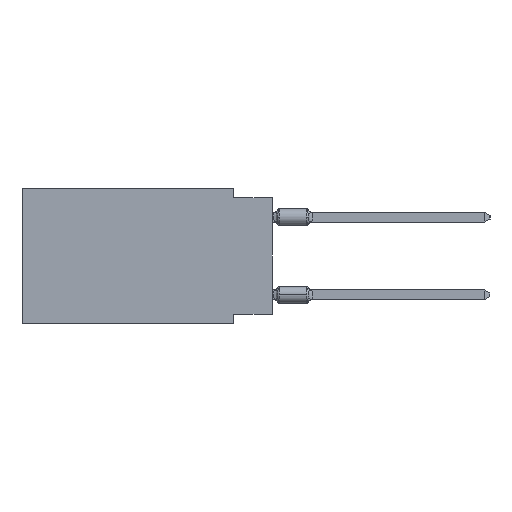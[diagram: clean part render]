
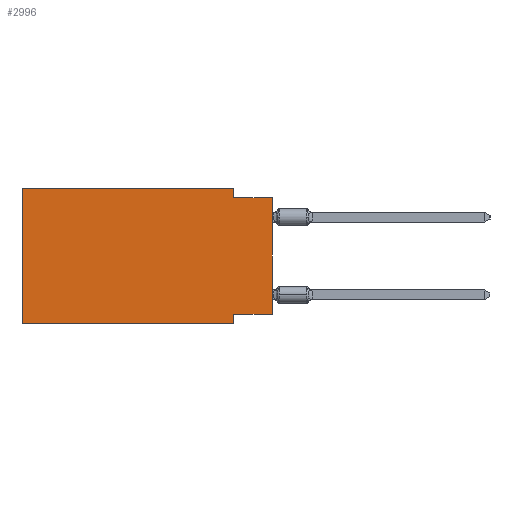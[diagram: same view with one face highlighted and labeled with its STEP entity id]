
A CAD part, left-side view. The second image highlights one B-rep face of the part: STEP entity #2996.
In plain terms, the highlighted planar face has unit normal (-1, 0, 0).
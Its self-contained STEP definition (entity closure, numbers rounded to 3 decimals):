
#128 = CARTESIAN_POINT ( 'NONE',  ( 0., 2.54, 0. ) ) ;
#219 = EDGE_CURVE ( 'NONE', #48608, #40719, #40505, .T. ) ;
#1783 = FACE_OUTER_BOUND ( 'NONE', #47971, .T. ) ;
#1838 = DIRECTION ( 'NONE',  ( 0., 0., 1. ) ) ;
#2594 = LINE ( 'NONE', #10689, #19937 ) ;
#2691 = LINE ( 'NONE', #21421, #8398 ) ;
#2996 = ADVANCED_FACE ( 'NONE', ( #1783 ), #17217, .F. ) ;
#3094 = DIRECTION ( 'NONE',  ( 0., -1., 0. ) ) ;
#3864 = ORIENTED_EDGE ( 'NONE', *, *, #18307, .F. ) ;
#4532 = VECTOR ( 'NONE', #36025, 1000. ) ;
#6313 = DIRECTION ( 'NONE',  ( 0., -1., 0. ) ) ;
#6457 = LINE ( 'NONE', #25908, #46648 ) ;
#6690 = VERTEX_POINT ( 'NONE', #7391 ) ;
#7211 = CARTESIAN_POINT ( 'NONE',  ( 0., 16.383, 0. ) ) ;
#7391 = CARTESIAN_POINT ( 'NONE',  ( 0., 2.54, -8.89 ) ) ;
#8398 = VECTOR ( 'NONE', #17646, 1000. ) ;
#9088 = CARTESIAN_POINT ( 'NONE',  ( 0., 0., -0.635 ) ) ;
#9103 = ORIENTED_EDGE ( 'NONE', *, *, #35650, .F. ) ;
#10689 = CARTESIAN_POINT ( 'NONE',  ( 0., 16.383, -8.89 ) ) ;
#11226 = DIRECTION ( 'NONE',  ( 0., 0., 1. ) ) ;
#11237 = VECTOR ( 'NONE', #15599, 1000. ) ;
#11817 = EDGE_CURVE ( 'NONE', #13317, #40719, #6457, .T. ) ;
#13317 = VERTEX_POINT ( 'NONE', #44213 ) ;
#13421 = DIRECTION ( 'NONE',  ( 0., 0., -1. ) ) ;
#14048 = VECTOR ( 'NONE', #6313, 1000. ) ;
#15599 = DIRECTION ( 'NONE',  ( 0., 1., 0. ) ) ;
#16341 = LINE ( 'NONE', #39072, #11237 ) ;
#17217 = PLANE ( 'NONE',  #43900 ) ;
#17646 = DIRECTION ( 'NONE',  ( 0., 0., -1. ) ) ;
#18307 = EDGE_CURVE ( 'NONE', #48608, #29607, #16341, .T. ) ;
#19371 = LINE ( 'NONE', #128, #4532 ) ;
#19937 = VECTOR ( 'NONE', #3094, 1000. ) ;
#21313 = CARTESIAN_POINT ( 'NONE',  ( 0., 0., 0. ) ) ;
#21421 = CARTESIAN_POINT ( 'NONE',  ( 0., 2.54, -8.89 ) ) ;
#21871 = DIRECTION ( 'NONE',  ( 0., -1., 0. ) ) ;
#23899 = ORIENTED_EDGE ( 'NONE', *, *, #45067, .F. ) ;
#24412 = ORIENTED_EDGE ( 'NONE', *, *, #219, .T. ) ;
#25908 = CARTESIAN_POINT ( 'NONE',  ( 0., 0., -0.635 ) ) ;
#26017 = CARTESIAN_POINT ( 'NONE',  ( 0., 2.54, 0. ) ) ;
#27883 = CARTESIAN_POINT ( 'NONE',  ( 0., 0., -8.255 ) ) ;
#28161 = ORIENTED_EDGE ( 'NONE', *, *, #43374, .F. ) ;
#29375 = EDGE_CURVE ( 'NONE', #40970, #6690, #2594, .T. ) ;
#29607 = VERTEX_POINT ( 'NONE', #39211 ) ;
#30298 = CARTESIAN_POINT ( 'NONE',  ( 0., 16.383, 0. ) ) ;
#32626 = CARTESIAN_POINT ( 'NONE',  ( 0., 16.383, 0. ) ) ;
#32643 = ORIENTED_EDGE ( 'NONE', *, *, #29375, .T. ) ;
#35650 = EDGE_CURVE ( 'NONE', #40171, #45871, #44947, .T. ) ;
#36025 = DIRECTION ( 'NONE',  ( 0., 0., -1. ) ) ;
#36143 = EDGE_CURVE ( 'NONE', #29607, #6690, #2691, .T. ) ;
#39072 = CARTESIAN_POINT ( 'NONE',  ( 0., 0., -8.255 ) ) ;
#39180 = ORIENTED_EDGE ( 'NONE', *, *, #11817, .F. ) ;
#39211 = CARTESIAN_POINT ( 'NONE',  ( 0., 2.54, -8.255 ) ) ;
#40171 = VERTEX_POINT ( 'NONE', #7211 ) ;
#40505 = LINE ( 'NONE', #21313, #41225 ) ;
#40719 = VERTEX_POINT ( 'NONE', #9088 ) ;
#40970 = VERTEX_POINT ( 'NONE', #42641 ) ;
#41225 = VECTOR ( 'NONE', #1838, 1000. ) ;
#42641 = CARTESIAN_POINT ( 'NONE',  ( 0., 16.383, -8.89 ) ) ;
#43374 = EDGE_CURVE ( 'NONE', #45871, #13317, #19371, .T. ) ;
#43900 = AXIS2_PLACEMENT_3D ( 'NONE', #32626, #48024, #13421 ) ;
#44213 = CARTESIAN_POINT ( 'NONE',  ( 0., 2.54, -0.635 ) ) ;
#44947 = LINE ( 'NONE', #30298, #14048 ) ;
#45067 = EDGE_CURVE ( 'NONE', #40970, #40171, #45815, .T. ) ;
#45293 = ORIENTED_EDGE ( 'NONE', *, *, #36143, .F. ) ;
#45815 = LINE ( 'NONE', #46069, #46305 ) ;
#45871 = VERTEX_POINT ( 'NONE', #26017 ) ;
#46069 = CARTESIAN_POINT ( 'NONE',  ( 0., 16.383, 0. ) ) ;
#46305 = VECTOR ( 'NONE', #11226, 1000. ) ;
#46648 = VECTOR ( 'NONE', #21871, 1000. ) ;
#47971 = EDGE_LOOP ( 'NONE', ( #24412, #39180, #28161, #9103, #23899, #32643, #45293, #3864 ) ) ;
#48024 = DIRECTION ( 'NONE',  ( 1., 0., 0. ) ) ;
#48608 = VERTEX_POINT ( 'NONE', #27883 ) ;
